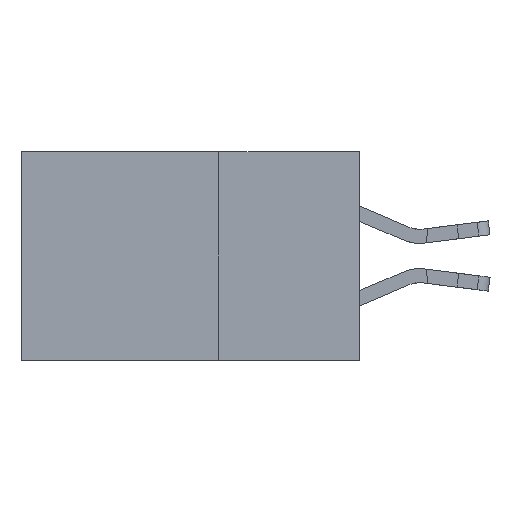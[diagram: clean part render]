
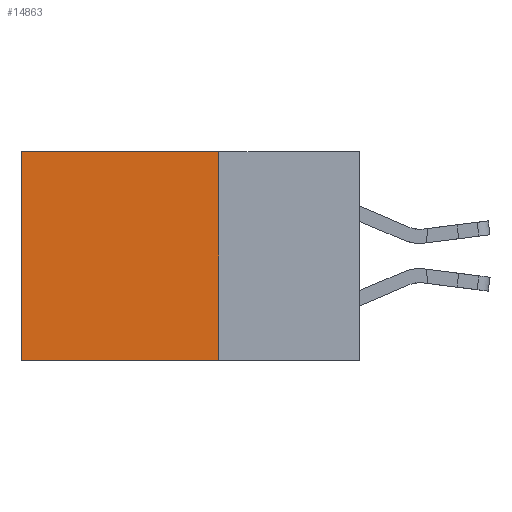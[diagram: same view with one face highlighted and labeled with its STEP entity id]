
A CAD part, left-side view. The second image highlights one B-rep face of the part: STEP entity #14863.
In plain terms, the highlighted planar face has unit normal (-1, 0, 0).
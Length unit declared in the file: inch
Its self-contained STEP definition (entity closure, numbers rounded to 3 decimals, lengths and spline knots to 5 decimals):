
#1009 = DIRECTION ( 'NONE',  ( 0., 1., 0. ) ) ;
#2171 = LINE ( 'NONE', #9643, #19794 ) ;
#2189 = EDGE_CURVE ( 'NONE', #22639, #22997, #2171, .T. ) ;
#2426 = DIRECTION ( 'NONE',  ( 0., 0., -1. ) ) ;
#3501 = CARTESIAN_POINT ( 'NONE',  ( 0.2875, 0.6, -0.37 ) ) ;
#4400 = LINE ( 'NONE', #20052, #26250 ) ;
#4723 = ORIENTED_EDGE ( 'NONE', *, *, #23138, .T. ) ;
#5053 = VECTOR ( 'NONE', #7819, 39.37008 ) ;
#6757 = EDGE_LOOP ( 'NONE', ( #10198, #25361, #21609, #4723 ) ) ;
#7473 = EDGE_CURVE ( 'NONE', #17627, #16762, #26223, .T. ) ;
#7819 = DIRECTION ( 'NONE',  ( 0., 0., -1. ) ) ;
#8001 = DIRECTION ( 'NONE',  ( 0., 1., 0. ) ) ;
#8816 = CARTESIAN_POINT ( 'NONE',  ( 0.2875, 0.25, 0. ) ) ;
#9548 = DIRECTION ( 'NONE',  ( 0., 0., -1. ) ) ;
#9559 = LINE ( 'NONE', #18556, #25760 ) ;
#9643 = CARTESIAN_POINT ( 'NONE',  ( 0.2875, 0.6, 0. ) ) ;
#10198 = ORIENTED_EDGE ( 'NONE', *, *, #2189, .T. ) ;
#10916 = CARTESIAN_POINT ( 'NONE',  ( 0.2875, 0.25, -0.37 ) ) ;
#13068 = CARTESIAN_POINT ( 'NONE',  ( 0.2875, 0.25, 0. ) ) ;
#14863 = ADVANCED_FACE ( 'NONE', ( #18947 ), #25709, .F. ) ;
#15211 = DIRECTION ( 'NONE',  ( 1., 0., 0. ) ) ;
#15732 = AXIS2_PLACEMENT_3D ( 'NONE', #13068, #15211, #2426 ) ;
#16762 = VERTEX_POINT ( 'NONE', #10916 ) ;
#17627 = VERTEX_POINT ( 'NONE', #8816 ) ;
#18556 = CARTESIAN_POINT ( 'NONE',  ( 0.2875, 0.25, 0. ) ) ;
#18947 = FACE_OUTER_BOUND ( 'NONE', #6757, .T. ) ;
#19794 = VECTOR ( 'NONE', #9548, 39.37008 ) ;
#20052 = CARTESIAN_POINT ( 'NONE',  ( 0.2875, 0.25, -0.37 ) ) ;
#20262 = EDGE_CURVE ( 'NONE', #16762, #22997, #4400, .T. ) ;
#21512 = CARTESIAN_POINT ( 'NONE',  ( 0.2875, 0.6, 0. ) ) ;
#21609 = ORIENTED_EDGE ( 'NONE', *, *, #7473, .F. ) ;
#22639 = VERTEX_POINT ( 'NONE', #21512 ) ;
#22997 = VERTEX_POINT ( 'NONE', #3501 ) ;
#23138 = EDGE_CURVE ( 'NONE', #17627, #22639, #9559, .T. ) ;
#24674 = CARTESIAN_POINT ( 'NONE',  ( 0.2875, 0.25, 0. ) ) ;
#25361 = ORIENTED_EDGE ( 'NONE', *, *, #20262, .F. ) ;
#25709 = PLANE ( 'NONE',  #15732 ) ;
#25760 = VECTOR ( 'NONE', #8001, 39.37008 ) ;
#26223 = LINE ( 'NONE', #24674, #5053 ) ;
#26250 = VECTOR ( 'NONE', #1009, 39.37008 ) ;
